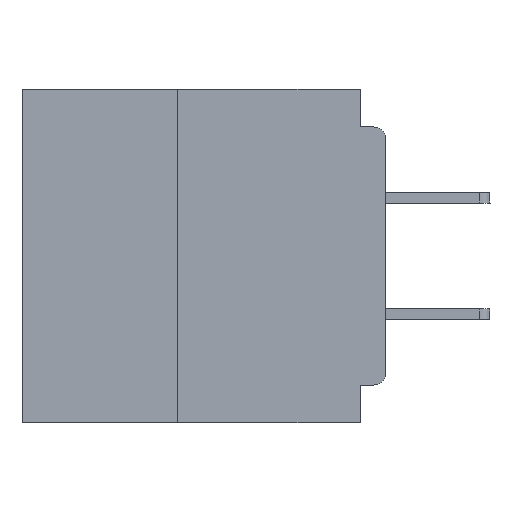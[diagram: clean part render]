
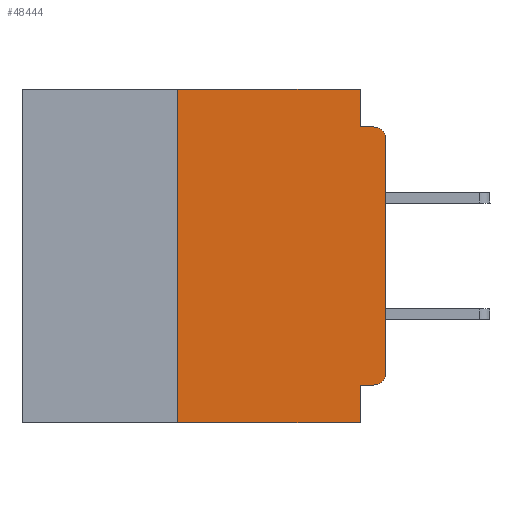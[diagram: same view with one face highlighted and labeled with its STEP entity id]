
A CAD part, left-side view. The second image highlights one B-rep face of the part: STEP entity #48444.
In plain terms, the highlighted planar face has unit normal (-1, 0, 0).
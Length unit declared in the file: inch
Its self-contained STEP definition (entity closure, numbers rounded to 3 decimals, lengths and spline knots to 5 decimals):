
#3636 = DIRECTION ( 'NONE',  ( 0., 0., 1. ) ) ;
#3823 = CARTESIAN_POINT ( 'NONE',  ( 0., 0.031, 0. ) ) ;
#4674 = VECTOR ( 'NONE', #32177, 39.37008 ) ;
#5123 = VECTOR ( 'NONE', #17631, 39.37008 ) ;
#5906 = VERTEX_POINT ( 'NONE', #46436 ) ;
#7214 = VECTOR ( 'NONE', #33727, 39.37008 ) ;
#8137 = VERTEX_POINT ( 'NONE', #64567 ) ;
#9455 = VERTEX_POINT ( 'NONE', #43922 ) ;
#9961 = VERTEX_POINT ( 'NONE', #26856 ) ;
#10349 = CARTESIAN_POINT ( 'NONE',  ( 0., 0.031, -0.355 ) ) ;
#12892 = AXIS2_PLACEMENT_3D ( 'NONE', #58178, #26738, #63462 ) ;
#13645 = LINE ( 'NONE', #35304, #41641 ) ;
#13990 = DIRECTION ( 'NONE',  ( 0., -1., 0. ) ) ;
#14221 = CARTESIAN_POINT ( 'NONE',  ( 0., 0.437, -0.4 ) ) ;
#14595 = ORIENTED_EDGE ( 'NONE', *, *, #47303, .F. ) ;
#16143 = PLANE ( 'NONE',  #12892 ) ;
#17571 = LINE ( 'NONE', #54351, #5123 ) ;
#17631 = DIRECTION ( 'NONE',  ( 0., 0., 1. ) ) ;
#17669 = VERTEX_POINT ( 'NONE', #61361 ) ;
#17827 = CARTESIAN_POINT ( 'NONE',  ( 0., 0., -0.045 ) ) ;
#18112 = EDGE_CURVE ( 'NONE', #9455, #34561, #49665, .T. ) ;
#18369 = ORIENTED_EDGE ( 'NONE', *, *, #25079, .F. ) ;
#18782 = LINE ( 'NONE', #63588, #4674 ) ;
#20491 = VERTEX_POINT ( 'NONE', #3823 ) ;
#21320 = LINE ( 'NONE', #17827, #7214 ) ;
#21700 = DIRECTION ( 'NONE',  ( 0., -1., 0. ) ) ;
#23803 = EDGE_CURVE ( 'NONE', #8137, #33166, #17571, .T. ) ;
#24651 = ORIENTED_EDGE ( 'NONE', *, *, #27244, .F. ) ;
#25079 = EDGE_CURVE ( 'NONE', #33166, #20491, #64239, .T. ) ;
#25292 = CARTESIAN_POINT ( 'NONE',  ( 0., 0., -0.06 ) ) ;
#26568 = DIRECTION ( 'NONE',  ( -1., 0., 0. ) ) ;
#26738 = DIRECTION ( 'NONE',  ( 1., 0., 0. ) ) ;
#26856 = CARTESIAN_POINT ( 'NONE',  ( 0., 0., -0.34 ) ) ;
#27244 = EDGE_CURVE ( 'NONE', #34561, #17669, #37679, .T. ) ;
#27975 = CIRCLE ( 'NONE', #49636, 0.015 ) ;
#28059 = CARTESIAN_POINT ( 'NONE',  ( 0., 0., -0.355 ) ) ;
#29997 = CARTESIAN_POINT ( 'NONE',  ( 0., 0.015, -0.34 ) ) ;
#32039 = CARTESIAN_POINT ( 'NONE',  ( 0., 0.437, 0. ) ) ;
#32177 = DIRECTION ( 'NONE',  ( 0., 0., -1. ) ) ;
#32435 = VERTEX_POINT ( 'NONE', #39093 ) ;
#33166 = VERTEX_POINT ( 'NONE', #56237 ) ;
#33727 = DIRECTION ( 'NONE',  ( 0., -1., 0. ) ) ;
#33895 = EDGE_CURVE ( 'NONE', #65776, #32435, #27975, .T. ) ;
#34561 = VERTEX_POINT ( 'NONE', #10349 ) ;
#35299 = DIRECTION ( 'NONE',  ( 0., 0., -1. ) ) ;
#35304 = CARTESIAN_POINT ( 'NONE',  ( 0., 0., 0. ) ) ;
#35784 = VECTOR ( 'NONE', #54387, 39.37008 ) ;
#37679 = LINE ( 'NONE', #55891, #63919 ) ;
#37973 = ORIENTED_EDGE ( 'NONE', *, *, #43129, .T. ) ;
#39093 = CARTESIAN_POINT ( 'NONE',  ( 0., 0.015, -0.045 ) ) ;
#40823 = FACE_OUTER_BOUND ( 'NONE', #57216, .T. ) ;
#41641 = VECTOR ( 'NONE', #3636, 39.37008 ) ;
#43129 = EDGE_CURVE ( 'NONE', #9455, #9961, #44763, .T. ) ;
#43922 = CARTESIAN_POINT ( 'NONE',  ( 0., 0.015, -0.355 ) ) ;
#44470 = ORIENTED_EDGE ( 'NONE', *, *, #52660, .T. ) ;
#44763 = CIRCLE ( 'NONE', #57065, 0.015 ) ;
#45613 = ORIENTED_EDGE ( 'NONE', *, *, #33895, .T. ) ;
#46436 = CARTESIAN_POINT ( 'NONE',  ( 0., 0.031, -0.045 ) ) ;
#47064 = EDGE_CURVE ( 'NONE', #5906, #32435, #21320, .T. ) ;
#47303 = EDGE_CURVE ( 'NONE', #20491, #5906, #18782, .T. ) ;
#47315 = LINE ( 'NONE', #14221, #59658 ) ;
#47429 = ORIENTED_EDGE ( 'NONE', *, *, #23803, .F. ) ;
#48444 = ADVANCED_FACE ( 'NONE', ( #40823 ), #16143, .F. ) ;
#49636 = AXIS2_PLACEMENT_3D ( 'NONE', #57991, #26568, #63294 ) ;
#49665 = LINE ( 'NONE', #28059, #35784 ) ;
#50230 = VECTOR ( 'NONE', #21700, 39.37008 ) ;
#52660 = EDGE_CURVE ( 'NONE', #9961, #65776, #13645, .T. ) ;
#54351 = CARTESIAN_POINT ( 'NONE',  ( 0., 0.25, -0.4 ) ) ;
#54387 = DIRECTION ( 'NONE',  ( 0., 1., 0. ) ) ;
#55891 = CARTESIAN_POINT ( 'NONE',  ( 0., 0.031, -0.4 ) ) ;
#56237 = CARTESIAN_POINT ( 'NONE',  ( 0., 0.25, 0. ) ) ;
#57065 = AXIS2_PLACEMENT_3D ( 'NONE', #29997, #66676, #35299 ) ;
#57216 = EDGE_LOOP ( 'NONE', ( #44470, #45613, #65490, #14595, #18369, #47429, #65925, #24651, #57552, #37973 ) ) ;
#57552 = ORIENTED_EDGE ( 'NONE', *, *, #18112, .F. ) ;
#57991 = CARTESIAN_POINT ( 'NONE',  ( 0., 0.015, -0.06 ) ) ;
#58178 = CARTESIAN_POINT ( 'NONE',  ( 0., 0.437, 0. ) ) ;
#59658 = VECTOR ( 'NONE', #13990, 39.37008 ) ;
#61191 = DIRECTION ( 'NONE',  ( 0., 0., -1. ) ) ;
#61361 = CARTESIAN_POINT ( 'NONE',  ( 0., 0.031, -0.4 ) ) ;
#62717 = EDGE_CURVE ( 'NONE', #8137, #17669, #47315, .T. ) ;
#63294 = DIRECTION ( 'NONE',  ( 0., 0., -1. ) ) ;
#63462 = DIRECTION ( 'NONE',  ( 0., 0., -1. ) ) ;
#63588 = CARTESIAN_POINT ( 'NONE',  ( 0., 0.031, 0. ) ) ;
#63919 = VECTOR ( 'NONE', #61191, 39.37008 ) ;
#64239 = LINE ( 'NONE', #32039, #50230 ) ;
#64567 = CARTESIAN_POINT ( 'NONE',  ( 0., 0.25, -0.4 ) ) ;
#65490 = ORIENTED_EDGE ( 'NONE', *, *, #47064, .F. ) ;
#65776 = VERTEX_POINT ( 'NONE', #25292 ) ;
#65925 = ORIENTED_EDGE ( 'NONE', *, *, #62717, .T. ) ;
#66676 = DIRECTION ( 'NONE',  ( -1., 0., 0. ) ) ;
